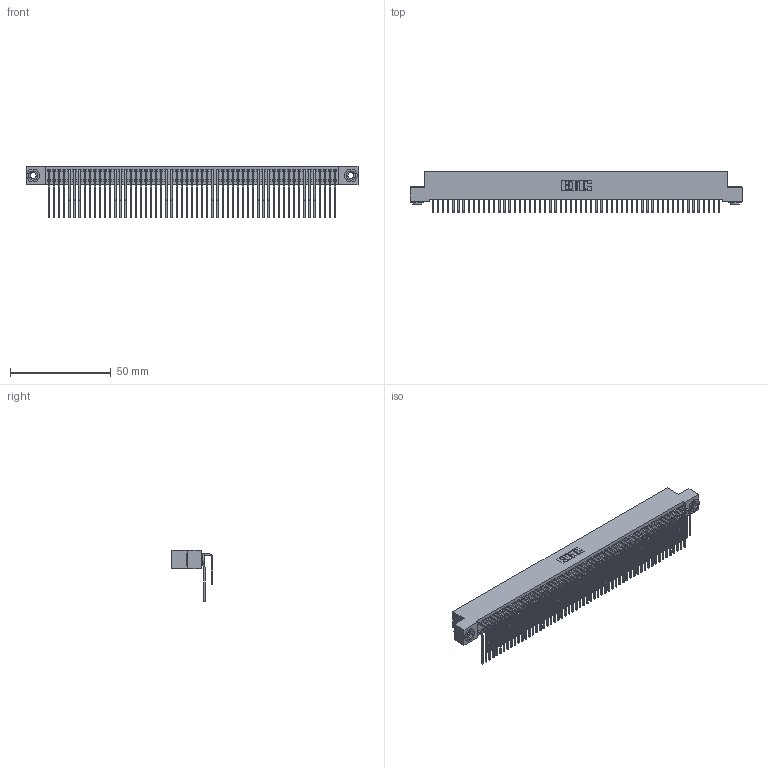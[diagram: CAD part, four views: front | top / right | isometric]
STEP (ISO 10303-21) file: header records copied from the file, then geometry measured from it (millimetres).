
FILE_DESCRIPTION (( 'STEP AP203' ), '1' );
FILE_NAME ('342-114-559-203.STEP', '2018-08-14T13:14:40', ( '' ), ( '' ), 'SwSTEP 2.0', 'SolidWorks 2016', '' );
FILE_SCHEMA (( 'CONFIG_CONTROL_DESIGN' ));
Length unit declared in the file: inch
Products named in the file (5): 342-114-559-203; 342 Part_.156 TH; 345-292-001_558 559 Tail - 1; 345-292-001_559 Tail - 2; 342-250-002_345-250-002-102
Assembly tree (117 placements, depth 2):
  342-114-559-203
    342 Part_.156 TH
    345-292-001_558 559 Tail - 1  x57
    345-292-001_559 Tail - 2  x57
    342-250-002_345-250-002-102  x2
Bounding box: 165.1 x 20.64 x 25.78 mm (x, y, z)
Volume: 15585.7 mm3; surface area: 28928.2 mm2
Topology: 117 solids, 117 shells, 6304 faces, 18729 edges, 12330 vertices
Faces by surface type: plane 4408, cylinder 1888, cone 8
Entity records: 37032 total; most frequent: CARTESIAN_POINT 6144, ORIENTED_EDGE 6022, DIRECTION 5237, EDGE_CURVE 3011, VECTOR 2819, LINE 2819, VERTEX_POINT 2002, AXIS2_PLACEMENT_3D 1209
